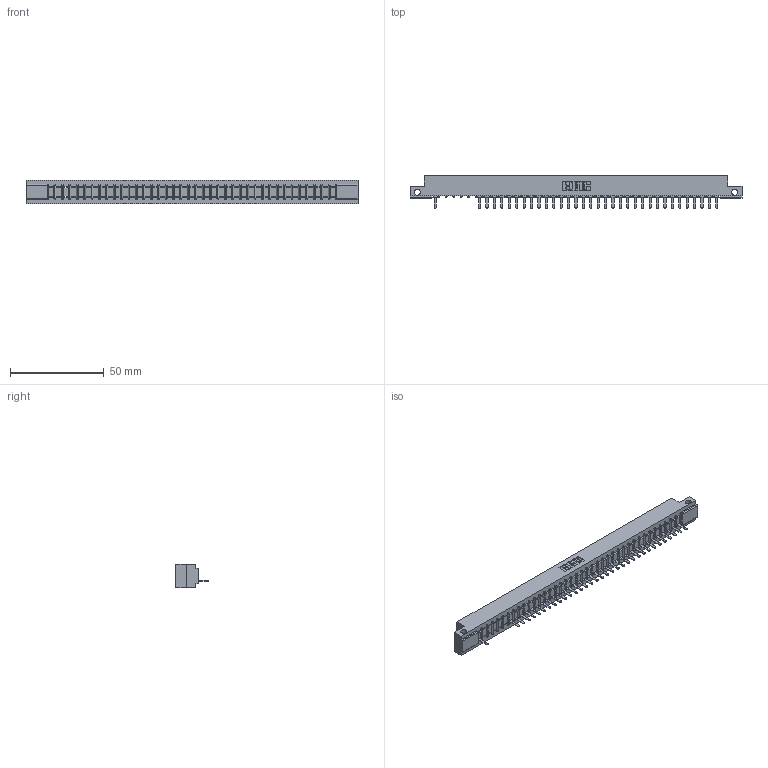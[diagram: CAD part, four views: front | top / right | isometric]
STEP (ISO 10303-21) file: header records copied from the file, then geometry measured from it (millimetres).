
FILE_DESCRIPTION (( 'STEP AP203' ), '1' );
FILE_NAME ('357-039-521-112.STEP', '2018-08-10T11:51:17', ( '' ), ( '' ), 'SwSTEP 2.0', 'SolidWorks 2016', '' );
FILE_SCHEMA (( 'CONFIG_CONTROL_DESIGN' ));
Length unit declared in the file: inch
Products named in the file (3): 307 Part_.128 Dia Side Mounting Holes; 307-290-002_521; 357-039-521-112
Assembly tree (35 placements, depth 2):
  357-039-521-112
    307 Part_.128 Dia Side Mounting Holes
    307-290-002_521  x34
Bounding box: 177.55 x 17.42 x 12.7 mm (x, y, z)
Volume: 18692.5 mm3; surface area: 22505.5 mm2
Topology: 35 solids, 35 shells, 2774 faces, 8531 edges, 5578 vertices
Faces by surface type: plane 1660, cylinder 1034, sphere 80
Entity records: 34364 total; most frequent: CARTESIAN_POINT 5819, ORIENTED_EDGE 5814, DIRECTION 5649, EDGE_CURVE 2907, LINE 2225, VECTOR 2225, VERTEX_POINT 1882, AXIS2_PLACEMENT_3D 1712
